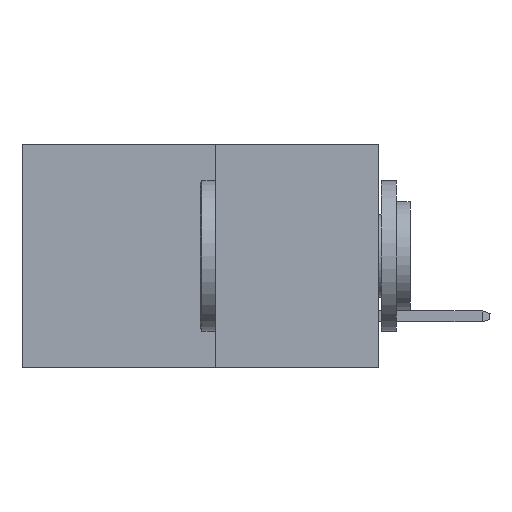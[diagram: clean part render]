
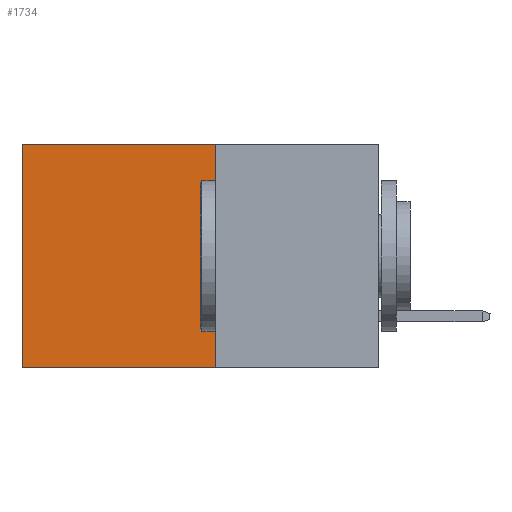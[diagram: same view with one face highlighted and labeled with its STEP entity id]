
A CAD part, left-side view. The second image highlights one B-rep face of the part: STEP entity #1734.
In plain terms, the highlighted planar face has unit normal (-1, 0, 0).
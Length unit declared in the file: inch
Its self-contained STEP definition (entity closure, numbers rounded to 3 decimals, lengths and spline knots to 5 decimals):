
#170 = VERTEX_POINT ( 'NONE', #5560 ) ;
#562 = LINE ( 'NONE', #10431, #11166 ) ;
#799 = CARTESIAN_POINT ( 'NONE',  ( 0.277, 0.59, 0. ) ) ;
#967 = VERTEX_POINT ( 'NONE', #1060 ) ;
#1060 = CARTESIAN_POINT ( 'NONE',  ( 0.277, 0.27, -0.37 ) ) ;
#1734 = ADVANCED_FACE ( 'NONE', ( #6207 ), #2752, .F. ) ;
#2006 = ORIENTED_EDGE ( 'NONE', *, *, #4066, .T. ) ;
#2008 = DIRECTION ( 'NONE',  ( 0., 1., 0. ) ) ;
#2300 = CARTESIAN_POINT ( 'NONE',  ( 0.277, 0.59, -0.37 ) ) ;
#2339 = ORIENTED_EDGE ( 'NONE', *, *, #2401, .F. ) ;
#2401 = EDGE_CURVE ( 'NONE', #5448, #967, #3231, .T. ) ;
#2752 = PLANE ( 'NONE',  #9515 ) ;
#3231 = LINE ( 'NONE', #13492, #8556 ) ;
#4066 = EDGE_CURVE ( 'NONE', #10441, #170, #6618, .T. ) ;
#5187 = ORIENTED_EDGE ( 'NONE', *, *, #13070, .T. ) ;
#5448 = VERTEX_POINT ( 'NONE', #11583 ) ;
#5560 = CARTESIAN_POINT ( 'NONE',  ( 0.277, 0.59, -0.37 ) ) ;
#5562 = DIRECTION ( 'NONE',  ( 1., 0., 0. ) ) ;
#5982 = LINE ( 'NONE', #8863, #11241 ) ;
#6207 = FACE_OUTER_BOUND ( 'NONE', #9845, .T. ) ;
#6617 = DIRECTION ( 'NONE',  ( 0., 0., -1. ) ) ;
#6618 = LINE ( 'NONE', #2300, #9134 ) ;
#7810 = DIRECTION ( 'NONE',  ( 0., 0., -1. ) ) ;
#8556 = VECTOR ( 'NONE', #7810, 39.37008 ) ;
#8863 = CARTESIAN_POINT ( 'NONE',  ( 0.277, 0.27, 0. ) ) ;
#9134 = VECTOR ( 'NONE', #10877, 39.37008 ) ;
#9515 = AXIS2_PLACEMENT_3D ( 'NONE', #10850, #5562, #6617 ) ;
#9845 = EDGE_LOOP ( 'NONE', ( #2006, #13149, #2339, #5187 ) ) ;
#9905 = DIRECTION ( 'NONE',  ( 0., 1., 0. ) ) ;
#10431 = CARTESIAN_POINT ( 'NONE',  ( 0.277, 0.27, -0.37 ) ) ;
#10441 = VERTEX_POINT ( 'NONE', #799 ) ;
#10850 = CARTESIAN_POINT ( 'NONE',  ( 0.277, 0.27, -0.37 ) ) ;
#10877 = DIRECTION ( 'NONE',  ( 0., 0., -1. ) ) ;
#11166 = VECTOR ( 'NONE', #2008, 39.37008 ) ;
#11241 = VECTOR ( 'NONE', #9905, 39.37008 ) ;
#11583 = CARTESIAN_POINT ( 'NONE',  ( 0.277, 0.27, 0. ) ) ;
#12229 = EDGE_CURVE ( 'NONE', #967, #170, #562, .T. ) ;
#13070 = EDGE_CURVE ( 'NONE', #5448, #10441, #5982, .T. ) ;
#13149 = ORIENTED_EDGE ( 'NONE', *, *, #12229, .F. ) ;
#13492 = CARTESIAN_POINT ( 'NONE',  ( 0.277, 0.27, -0.37 ) ) ;
